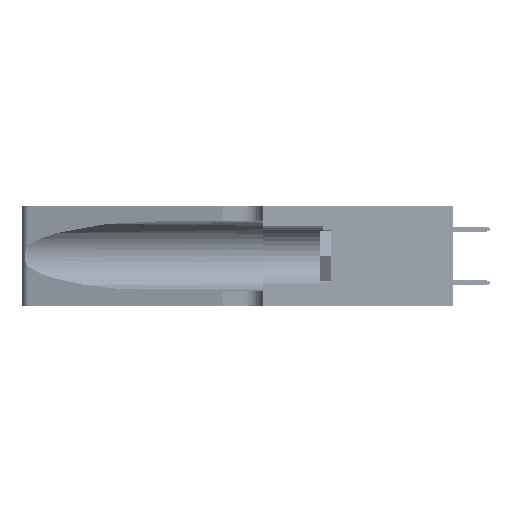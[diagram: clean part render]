
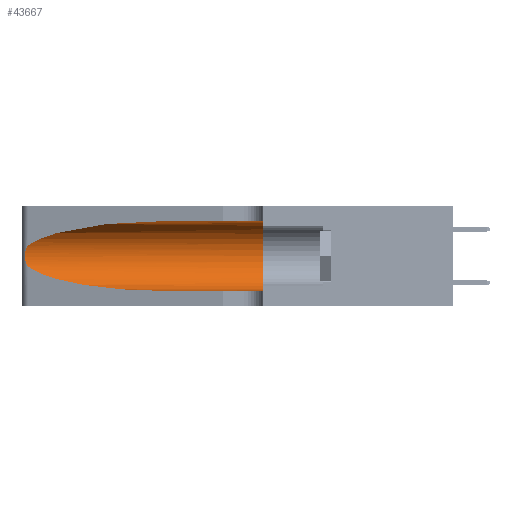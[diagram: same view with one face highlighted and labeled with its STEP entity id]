
A CAD part, left-side view. The second image highlights one B-rep face of the part: STEP entity #43667.
In plain terms, the highlighted cylindrical face has radius 3.308 mm (diameter 6.617 mm), a partial arc.
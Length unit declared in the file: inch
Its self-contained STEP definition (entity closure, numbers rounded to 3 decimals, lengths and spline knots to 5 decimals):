
#382 = EDGE_LOOP ( 'NONE', ( #743, #18124, #41837, #41783, #45200, #15470 ) ) ;
#743 = ORIENTED_EDGE ( 'NONE', *, *, #13120, .T. ) ;
#1259 = CYLINDRICAL_SURFACE ( 'NONE', #36742, 0.13025 ) ;
#2711 = CARTESIAN_POINT ( 'NONE',  ( 0.25555, 1.22994, 0.2215 ) ) ;
#2973 = CARTESIAN_POINT ( 'NONE',  ( 0.25487, 1.22718, 0.14631 ) ) ;
#3727 = VERTEX_POINT ( 'NONE', #17031 ) ;
#3915 = VECTOR ( 'NONE', #48258, 39.37008 ) ;
#4158 = CARTESIAN_POINT ( 'NONE',  ( 0.1305, 1.61858, 0.31525 ) ) ;
#5274 = AXIS2_PLACEMENT_3D ( 'NONE', #13760, #48997, #16950 ) ;
#5314 = EDGE_CURVE ( 'NONE', #47675, #29439, #52212, .T. ) ;
#5639 = CARTESIAN_POINT ( 'NONE',  ( 0.1305, 0.72297, 0.31525 ) ) ;
#7199 = CARTESIAN_POINT ( 'NONE',  ( 0.25487, 1.22718, 0.22369 ) ) ;
#7463 = CARTESIAN_POINT ( 'NONE',  ( 0.26075, 1.23896, 0.19203 ) ) ;
#7760 = VECTOR ( 'NONE', #20560, 39.37008 ) ;
#8234 = EDGE_CURVE ( 'NONE', #3727, #49870, #26285, .T. ) ;
#8649 = CIRCLE ( 'NONE', #5274, 0.13025 ) ;
#9198 = CARTESIAN_POINT ( 'NONE',  ( 0.25487, 1.22718, 0.14631 ) ) ;
#11448 = CARTESIAN_POINT ( 'NONE',  ( 0.1305, 0.35, 0.31525 ) ) ;
#13120 = EDGE_CURVE ( 'NONE', #48025, #3727, #44119, .T. ) ;
#13760 = CARTESIAN_POINT ( 'NONE',  ( 0.1305, 0.35, 0.185 ) ) ;
#14246 = EDGE_CURVE ( 'NONE', #48025, #41348, #40397, .T. ) ;
#14608 = CARTESIAN_POINT ( 'NONE',  ( 0.26018, 1.23835, 0.19895 ) ) ;
#14866 = CARTESIAN_POINT ( 'NONE',  ( 0.26075, 1.23896, 0.178 ) ) ;
#15470 = ORIENTED_EDGE ( 'NONE', *, *, #14246, .F. ) ;
#15947 = CARTESIAN_POINT ( 'NONE',  ( 0.1305, 1.61858, 0.05475 ) ) ;
#16950 = DIRECTION ( 'NONE',  ( 0., 0., 1. ) ) ;
#17031 = CARTESIAN_POINT ( 'NONE',  ( 0.25487, 1.22718, 0.22369 ) ) ;
#17142 = DIRECTION ( 'NONE',  ( 0., -1., 0. ) ) ;
#18079 = CARTESIAN_POINT ( 'NONE',  ( 0.18966, 0.96281, 0.31525 ) ) ;
#18106 = CARTESIAN_POINT ( 'NONE',  ( 0.25487, 1.22718, 0.14631 ) ) ;
#18124 = ORIENTED_EDGE ( 'NONE', *, *, #8234, .T. ) ;
#20560 = DIRECTION ( 'NONE',  ( 0., -1., 0. ) ) ;
#22474 = CARTESIAN_POINT ( 'NONE',  ( 0.1305, 0.35, 0.05475 ) ) ;
#26285 = B_SPLINE_CURVE_WITH_KNOTS ( 'NONE', 3,
 ( #7199, #2711, #38684, #39219, #31544, #14608, #7463, #14866, #35507, #31021, #27332, #30766, #46897, #2973 ),
 .UNSPECIFIED., .F., .F.,
 ( 4, 2, 2, 2, 2, 2, 4 ),
 ( 0., 0.00027, 0.00053, 0.00107, 0.0016, 0.00187, 0.00214 ),
 .UNSPECIFIED. ) ;
#26573 = CARTESIAN_POINT ( 'NONE',  ( 0.2373, 1.15595, 0.08982 ) ) ;
#27156 = EDGE_CURVE ( 'NONE', #49870, #47675, #49531, .T. ) ;
#27332 = CARTESIAN_POINT ( 'NONE',  ( 0.25789, 1.23486, 0.15765 ) ) ;
#29313 = CARTESIAN_POINT ( 'NONE',  ( 0.1305, 1.61858, 0.185 ) ) ;
#29439 = VERTEX_POINT ( 'NONE', #22474 ) ;
#30531 = EDGE_CURVE ( 'NONE', #41348, #29439, #8649, .T. ) ;
#30766 = CARTESIAN_POINT ( 'NONE',  ( 0.25639, 1.23186, 0.15144 ) ) ;
#31021 = CARTESIAN_POINT ( 'NONE',  ( 0.25856, 1.23593, 0.16098 ) ) ;
#31544 = CARTESIAN_POINT ( 'NONE',  ( 0.25854, 1.2359, 0.20912 ) ) ;
#32543 = CARTESIAN_POINT ( 'NONE',  ( 0.1305, 0.72297, 0.05475 ) ) ;
#33953 = CARTESIAN_POINT ( 'NONE',  ( 0.1305, 0.72297, 0.31525 ) ) ;
#35507 = CARTESIAN_POINT ( 'NONE',  ( 0.26017, 1.23833, 0.17102 ) ) ;
#36742 = AXIS2_PLACEMENT_3D ( 'NONE', #29313, #17142, #41216 ) ;
#37391 = CARTESIAN_POINT ( 'NONE',  ( 0.2373, 1.15595, 0.28018 ) ) ;
#37495 = FACE_OUTER_BOUND ( 'NONE', #382, .T. ) ;
#38684 = CARTESIAN_POINT ( 'NONE',  ( 0.25639, 1.23184, 0.21858 ) ) ;
#39219 = CARTESIAN_POINT ( 'NONE',  ( 0.25787, 1.23484, 0.2124 ) ) ;
#40397 = LINE ( 'NONE', #4158, #7760 ) ;
#41216 = DIRECTION ( 'NONE',  ( 0., 0., -1. ) ) ;
#41348 = VERTEX_POINT ( 'NONE', #11448 ) ;
#41783 = ORIENTED_EDGE ( 'NONE', *, *, #5314, .T. ) ;
#41837 = ORIENTED_EDGE ( 'NONE', *, *, #27156, .T. ) ;
#42444 = CARTESIAN_POINT ( 'NONE',  ( 0.1305, 0.72297, 0.05475 ) ) ;
#43667 = ADVANCED_FACE ( 'NONE', ( #37495 ), #1259, .F. ) ;
#44119 =( BOUNDED_CURVE ( )  B_SPLINE_CURVE ( 3, ( #5639, #18079, #37391, #46380 ),
 .UNSPECIFIED., .F., .T. ) 
 B_SPLINE_CURVE_WITH_KNOTS ( ( 4, 4 ),
 ( 1.5708, 2.84003 ),
 .UNSPECIFIED. ) 
 CURVE ( )  GEOMETRIC_REPRESENTATION_ITEM ( )  RATIONAL_B_SPLINE_CURVE ( ( 1., 0.87, 0.87, 1. ) ) 
 REPRESENTATION_ITEM ( '' )  );
#45200 = ORIENTED_EDGE ( 'NONE', *, *, #30531, .F. ) ;
#46380 = CARTESIAN_POINT ( 'NONE',  ( 0.25487, 1.22718, 0.22369 ) ) ;
#46897 = CARTESIAN_POINT ( 'NONE',  ( 0.25555, 1.22993, 0.14849 ) ) ;
#46922 = CARTESIAN_POINT ( 'NONE',  ( 0.18966, 0.96281, 0.05475 ) ) ;
#47675 = VERTEX_POINT ( 'NONE', #32543 ) ;
#48025 = VERTEX_POINT ( 'NONE', #33953 ) ;
#48258 = DIRECTION ( 'NONE',  ( 0., -1., 0. ) ) ;
#48997 = DIRECTION ( 'NONE',  ( 0., 1., 0. ) ) ;
#49531 =( BOUNDED_CURVE ( )  B_SPLINE_CURVE ( 3, ( #18106, #26573, #46922, #42444 ),
 .UNSPECIFIED., .F., .F. ) 
 B_SPLINE_CURVE_WITH_KNOTS ( ( 4, 4 ),
 ( 3.44316, 4.71239 ),
 .UNSPECIFIED. ) 
 CURVE ( )  GEOMETRIC_REPRESENTATION_ITEM ( )  RATIONAL_B_SPLINE_CURVE ( ( 1., 0.87, 0.87, 1. ) ) 
 REPRESENTATION_ITEM ( '' )  );
#49870 = VERTEX_POINT ( 'NONE', #9198 ) ;
#52212 = LINE ( 'NONE', #15947, #3915 ) ;
